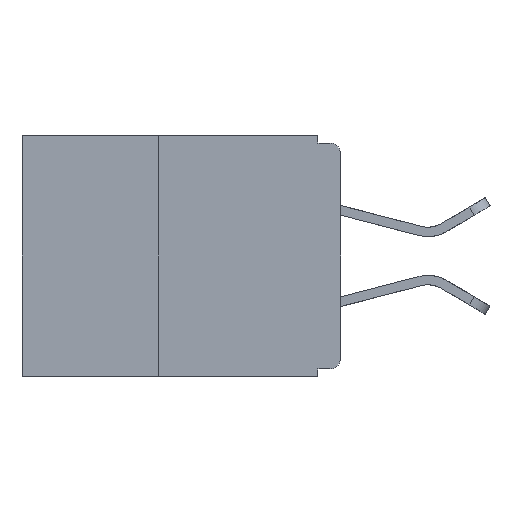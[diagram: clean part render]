
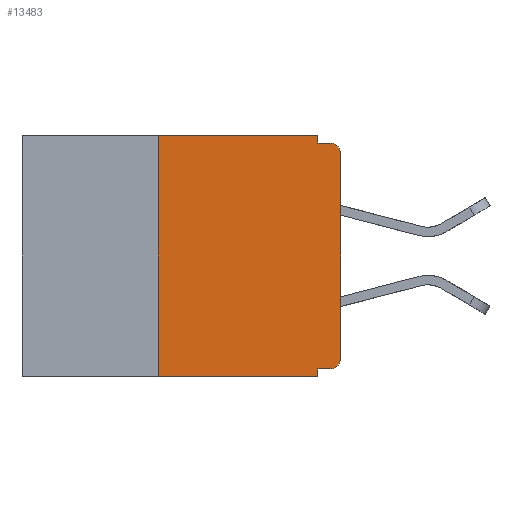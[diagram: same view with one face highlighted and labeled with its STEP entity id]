
A CAD part, left-side view. The second image highlights one B-rep face of the part: STEP entity #13483.
In plain terms, the highlighted planar face has unit normal (-1, 0, 0).
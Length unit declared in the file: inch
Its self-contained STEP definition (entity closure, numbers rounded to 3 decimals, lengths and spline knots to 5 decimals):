
#2 = VECTOR ( 'NONE', #2778, 39.37008 ) ;
#503 = CARTESIAN_POINT ( 'NONE',  ( 0., 0.015, -0.01 ) ) ;
#1154 = VERTEX_POINT ( 'NONE', #9988 ) ;
#1162 = LINE ( 'NONE', #3528, #22748 ) ;
#1402 = VERTEX_POINT ( 'NONE', #10775 ) ;
#1554 = VECTOR ( 'NONE', #12149, 39.37008 ) ;
#1971 = DIRECTION ( 'NONE',  ( 0., -1., 0. ) ) ;
#2728 = CIRCLE ( 'NONE', #14575, 0.015 ) ;
#2771 = CARTESIAN_POINT ( 'NONE',  ( 0., 0., -0.01 ) ) ;
#2778 = DIRECTION ( 'NONE',  ( 0., 0., 1. ) ) ;
#2948 = DIRECTION ( 'NONE',  ( 0., 0., -1. ) ) ;
#3370 = CARTESIAN_POINT ( 'NONE',  ( 0., 0.015, -0.305 ) ) ;
#3413 = DIRECTION ( 'NONE',  ( 0., 1., 0. ) ) ;
#3497 = LINE ( 'NONE', #23450, #22754 ) ;
#3499 = CIRCLE ( 'NONE', #7980, 0.015 ) ;
#3528 = CARTESIAN_POINT ( 'NONE',  ( 0., 0., -0.32 ) ) ;
#3816 = VERTEX_POINT ( 'NONE', #7955 ) ;
#4640 = FACE_OUTER_BOUND ( 'NONE', #23218, .T. ) ;
#5351 = AXIS2_PLACEMENT_3D ( 'NONE', #30381, #17962, #2948 ) ;
#5606 = CARTESIAN_POINT ( 'NONE',  ( 0., 0.25, 0. ) ) ;
#5856 = CARTESIAN_POINT ( 'NONE',  ( 0., 0.031, -0.33 ) ) ;
#5941 = DIRECTION ( 'NONE',  ( 0., 0., -1. ) ) ;
#6348 = DIRECTION ( 'NONE',  ( -1., 0., 0. ) ) ;
#6378 = CARTESIAN_POINT ( 'NONE',  ( 0., 0.015, -0.32 ) ) ;
#7010 = ORIENTED_EDGE ( 'NONE', *, *, #8287, .F. ) ;
#7473 = LINE ( 'NONE', #22855, #2 ) ;
#7955 = CARTESIAN_POINT ( 'NONE',  ( 0., 0.031, 0. ) ) ;
#7980 = AXIS2_PLACEMENT_3D ( 'NONE', #3370, #20890, #5941 ) ;
#8272 = LINE ( 'NONE', #19544, #1554 ) ;
#8287 = EDGE_CURVE ( 'NONE', #23050, #14673, #21889, .T. ) ;
#8430 = EDGE_CURVE ( 'NONE', #23308, #1154, #17941, .T. ) ;
#9988 = CARTESIAN_POINT ( 'NONE',  ( 0., 0.031, -0.33 ) ) ;
#10775 = CARTESIAN_POINT ( 'NONE',  ( 0., 0., -0.305 ) ) ;
#11057 = CARTESIAN_POINT ( 'NONE',  ( 0., 0.031, -0.01 ) ) ;
#11283 = VECTOR ( 'NONE', #29401, 39.37008 ) ;
#11327 = VECTOR ( 'NONE', #20822, 39.37008 ) ;
#11757 = EDGE_CURVE ( 'NONE', #31569, #1154, #3497, .T. ) ;
#12149 = DIRECTION ( 'NONE',  ( 0., 0., 1. ) ) ;
#12424 = EDGE_CURVE ( 'NONE', #25987, #14673, #2728, .T. ) ;
#12959 = PLANE ( 'NONE',  #5351 ) ;
#13091 = LINE ( 'NONE', #26937, #18902 ) ;
#13303 = ORIENTED_EDGE ( 'NONE', *, *, #8430, .F. ) ;
#13483 = ADVANCED_FACE ( 'NONE', ( #4640 ), #12959, .F. ) ;
#13853 = CARTESIAN_POINT ( 'NONE',  ( 0., 0., -0.025 ) ) ;
#14385 = CARTESIAN_POINT ( 'NONE',  ( 0., 0.031, 0. ) ) ;
#14575 = AXIS2_PLACEMENT_3D ( 'NONE', #21303, #6348, #23861 ) ;
#14673 = VERTEX_POINT ( 'NONE', #503 ) ;
#15251 = VECTOR ( 'NONE', #27838, 39.37008 ) ;
#15652 = ORIENTED_EDGE ( 'NONE', *, *, #31394, .T. ) ;
#16021 = ORIENTED_EDGE ( 'NONE', *, *, #20371, .F. ) ;
#16775 = EDGE_CURVE ( 'NONE', #31569, #31333, #8272, .T. ) ;
#17584 = ORIENTED_EDGE ( 'NONE', *, *, #11757, .T. ) ;
#17896 = LINE ( 'NONE', #14385, #11283 ) ;
#17941 = LINE ( 'NONE', #5856, #11327 ) ;
#17962 = DIRECTION ( 'NONE',  ( 1., 0., 0. ) ) ;
#18431 = EDGE_CURVE ( 'NONE', #3816, #23050, #17896, .T. ) ;
#18902 = VECTOR ( 'NONE', #1971, 39.37008 ) ;
#19544 = CARTESIAN_POINT ( 'NONE',  ( 0., 0.25, -0.33 ) ) ;
#20286 = ORIENTED_EDGE ( 'NONE', *, *, #18431, .F. ) ;
#20371 = EDGE_CURVE ( 'NONE', #31333, #3816, #13091, .T. ) ;
#20822 = DIRECTION ( 'NONE',  ( 0., 0., -1. ) ) ;
#20890 = DIRECTION ( 'NONE',  ( -1., 0., 0. ) ) ;
#21303 = CARTESIAN_POINT ( 'NONE',  ( 0., 0.015, -0.025 ) ) ;
#21889 = LINE ( 'NONE', #2771, #15251 ) ;
#22748 = VECTOR ( 'NONE', #3413, 39.37008 ) ;
#22754 = VECTOR ( 'NONE', #25940, 39.37008 ) ;
#22855 = CARTESIAN_POINT ( 'NONE',  ( 0., 0., 0. ) ) ;
#23050 = VERTEX_POINT ( 'NONE', #11057 ) ;
#23218 = EDGE_LOOP ( 'NONE', ( #31949, #26180, #7010, #20286, #16021, #30038, #17584, #13303, #26590, #15652 ) ) ;
#23308 = VERTEX_POINT ( 'NONE', #29528 ) ;
#23450 = CARTESIAN_POINT ( 'NONE',  ( 0., 0.437, -0.33 ) ) ;
#23861 = DIRECTION ( 'NONE',  ( 0., 0., -1. ) ) ;
#23993 = CARTESIAN_POINT ( 'NONE',  ( 0., 0.25, -0.33 ) ) ;
#25940 = DIRECTION ( 'NONE',  ( 0., -1., 0. ) ) ;
#25987 = VERTEX_POINT ( 'NONE', #13853 ) ;
#26180 = ORIENTED_EDGE ( 'NONE', *, *, #12424, .T. ) ;
#26590 = ORIENTED_EDGE ( 'NONE', *, *, #30798, .F. ) ;
#26937 = CARTESIAN_POINT ( 'NONE',  ( 0., 0.437, 0. ) ) ;
#27838 = DIRECTION ( 'NONE',  ( 0., -1., 0. ) ) ;
#29401 = DIRECTION ( 'NONE',  ( 0., 0., -1. ) ) ;
#29528 = CARTESIAN_POINT ( 'NONE',  ( 0., 0.031, -0.32 ) ) ;
#30038 = ORIENTED_EDGE ( 'NONE', *, *, #16775, .F. ) ;
#30381 = CARTESIAN_POINT ( 'NONE',  ( 0., 0.437, 0. ) ) ;
#30609 = EDGE_CURVE ( 'NONE', #1402, #25987, #7473, .T. ) ;
#30798 = EDGE_CURVE ( 'NONE', #31526, #23308, #1162, .T. ) ;
#31333 = VERTEX_POINT ( 'NONE', #5606 ) ;
#31394 = EDGE_CURVE ( 'NONE', #31526, #1402, #3499, .T. ) ;
#31526 = VERTEX_POINT ( 'NONE', #6378 ) ;
#31569 = VERTEX_POINT ( 'NONE', #23993 ) ;
#31949 = ORIENTED_EDGE ( 'NONE', *, *, #30609, .T. ) ;
